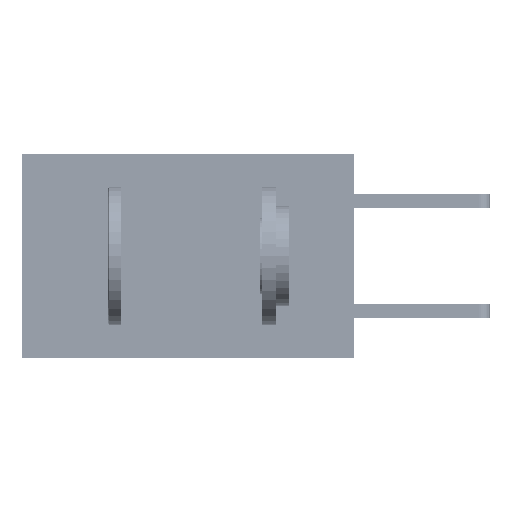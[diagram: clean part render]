
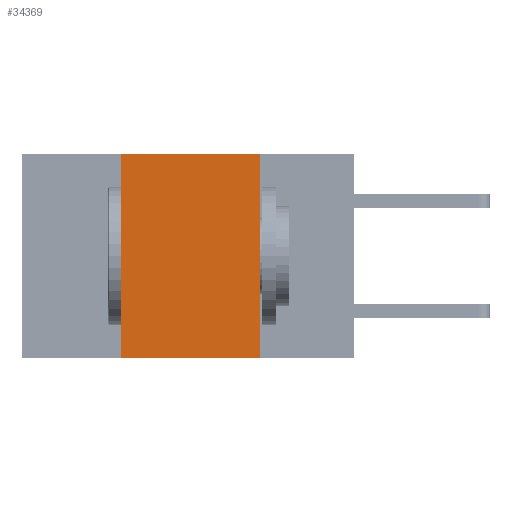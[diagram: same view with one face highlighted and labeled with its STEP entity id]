
A CAD part, left-side view. The second image highlights one B-rep face of the part: STEP entity #34369.
In plain terms, the highlighted planar face has unit normal (-1, 0, 0).
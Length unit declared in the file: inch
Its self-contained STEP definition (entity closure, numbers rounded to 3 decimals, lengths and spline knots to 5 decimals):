
#1428 = DIRECTION ( 'NONE',  ( 0., 0., -1. ) ) ;
#1456 = EDGE_CURVE ( 'NONE', #30193, #16569, #41097, .T. ) ;
#3358 = FACE_OUTER_BOUND ( 'NONE', #6255, .T. ) ;
#4941 = CARTESIAN_POINT ( 'NONE',  ( 0., 0.42, 0. ) ) ;
#5097 = CARTESIAN_POINT ( 'NONE',  ( 0., 0.6, 0. ) ) ;
#6255 = EDGE_LOOP ( 'NONE', ( #34501, #28407, #38851, #37534 ) ) ;
#8612 = VECTOR ( 'NONE', #17902, 39.37008 ) ;
#9912 = CARTESIAN_POINT ( 'NONE',  ( 0., 0.42, -0.37 ) ) ;
#15781 = VECTOR ( 'NONE', #20517, 39.37008 ) ;
#16569 = VERTEX_POINT ( 'NONE', #30106 ) ;
#17902 = DIRECTION ( 'NONE',  ( 0., 0., 1. ) ) ;
#19956 = DIRECTION ( 'NONE',  ( 0., -1., 0. ) ) ;
#20517 = DIRECTION ( 'NONE',  ( 0., 0., -1. ) ) ;
#20587 = EDGE_CURVE ( 'NONE', #16569, #20741, #25258, .T. ) ;
#20741 = VERTEX_POINT ( 'NONE', #40116 ) ;
#21676 = CARTESIAN_POINT ( 'NONE',  ( 0., 0.6, 0. ) ) ;
#24179 = AXIS2_PLACEMENT_3D ( 'NONE', #5097, #41358, #1428 ) ;
#25258 = LINE ( 'NONE', #32384, #15781 ) ;
#26054 = EDGE_CURVE ( 'NONE', #31299, #30193, #32353, .T. ) ;
#26315 = VECTOR ( 'NONE', #19956, 39.37008 ) ;
#28407 = ORIENTED_EDGE ( 'NONE', *, *, #1456, .F. ) ;
#29390 = EDGE_CURVE ( 'NONE', #31299, #20741, #36207, .T. ) ;
#30106 = CARTESIAN_POINT ( 'NONE',  ( 0., 0.17, 0. ) ) ;
#30193 = VERTEX_POINT ( 'NONE', #30679 ) ;
#30679 = CARTESIAN_POINT ( 'NONE',  ( 0., 0.42, 0. ) ) ;
#31299 = VERTEX_POINT ( 'NONE', #9912 ) ;
#32353 = LINE ( 'NONE', #4941, #8612 ) ;
#32384 = CARTESIAN_POINT ( 'NONE',  ( 0., 0.17, 0. ) ) ;
#33277 = VECTOR ( 'NONE', #34099, 39.37008 ) ;
#34099 = DIRECTION ( 'NONE',  ( 0., -1., 0. ) ) ;
#34369 = ADVANCED_FACE ( 'NONE', ( #3358 ), #38194, .F. ) ;
#34501 = ORIENTED_EDGE ( 'NONE', *, *, #20587, .F. ) ;
#36166 = CARTESIAN_POINT ( 'NONE',  ( 0., 0.6, -0.37 ) ) ;
#36207 = LINE ( 'NONE', #36166, #26315 ) ;
#37534 = ORIENTED_EDGE ( 'NONE', *, *, #29390, .T. ) ;
#38194 = PLANE ( 'NONE',  #24179 ) ;
#38851 = ORIENTED_EDGE ( 'NONE', *, *, #26054, .F. ) ;
#40116 = CARTESIAN_POINT ( 'NONE',  ( 0., 0.17, -0.37 ) ) ;
#41097 = LINE ( 'NONE', #21676, #33277 ) ;
#41358 = DIRECTION ( 'NONE',  ( 1., 0., 0. ) ) ;
